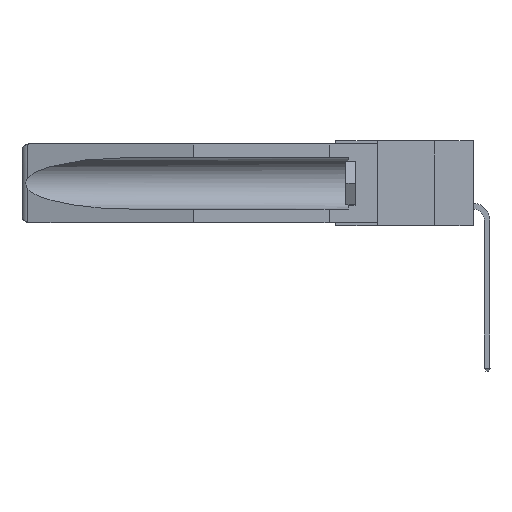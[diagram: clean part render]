
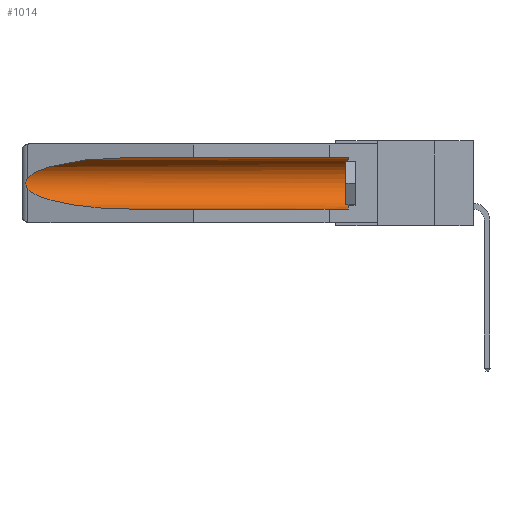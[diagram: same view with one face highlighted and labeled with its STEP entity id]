
A CAD part, left-side view. The second image highlights one B-rep face of the part: STEP entity #1014.
In plain terms, the highlighted cylindrical face has radius 2.857 mm (diameter 5.715 mm), a partial arc.
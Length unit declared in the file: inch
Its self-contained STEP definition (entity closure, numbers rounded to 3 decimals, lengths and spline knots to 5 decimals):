
#1 = EDGE_CURVE ( 'NONE', #16798, #9461, #5213, .T. ) ;
#342 = EDGE_CURVE ( 'NONE', #28409, #3035, #25971, .T. ) ;
#421 = CARTESIAN_POINT ( 'NONE',  ( 0.26597, 1.52961, -0.15275 ) ) ;
#663 = CARTESIAN_POINT ( 'NONE',  ( 0.155, -0.30754, -0.284 ) ) ;
#749 = CARTESIAN_POINT ( 'NONE',  ( 0.26655, 1.53094, -0.18657 ) ) ;
#1014 = ADVANCED_FACE ( 'NONE', ( #7717 ), #3617, .F. ) ;
#2842 = VERTEX_POINT ( 'NONE', #23426 ) ;
#3035 = VERTEX_POINT ( 'NONE', #10292 ) ;
#3096 = DIRECTION ( 'NONE',  ( 0., 1., 0. ) ) ;
#3443 = CARTESIAN_POINT ( 'NONE',  ( 0.155, 0.126, -0.1715 ) ) ;
#3617 = CYLINDRICAL_SURFACE ( 'NONE', #13320, 0.1125 ) ;
#3730 = VERTEX_POINT ( 'NONE', #18073 ) ;
#3817 = CARTESIAN_POINT ( 'NONE',  ( 0.155, 1.07973, -0.284 ) ) ;
#4316 = CARTESIAN_POINT ( 'NONE',  ( 0.26537, 1.52718, -0.14972 ) ) ;
#4538 = CARTESIAN_POINT ( 'NONE',  ( 0.155, 1.07973, -0.284 ) ) ;
#4825 =( BOUNDED_CURVE ( )  B_SPLINE_CURVE ( 3, ( #25880, #23379, #13919, #4316 ),
 .UNSPECIFIED., .F., .F. ) 
 B_SPLINE_CURVE_WITH_KNOTS ( ( 4, 4 ),
 ( 4.71239, 6.08839 ),
 .UNSPECIFIED. ) 
 CURVE ( )  GEOMETRIC_REPRESENTATION_ITEM ( )  RATIONAL_B_SPLINE_CURVE ( ( 1., 0.848, 0.848, 1. ) ) 
 REPRESENTATION_ITEM ( '' )  );
#5213 = LINE ( 'NONE', #663, #25657 ) ;
#6228 = CIRCLE ( 'NONE', #29589, 0.1125 ) ;
#7695 = EDGE_LOOP ( 'NONE', ( #25274, #15216, #8039, #23399, #27184, #23420 ) ) ;
#7717 = FACE_OUTER_BOUND ( 'NONE', #7695, .T. ) ;
#8039 = ORIENTED_EDGE ( 'NONE', *, *, #24191, .T. ) ;
#8237 = DIRECTION ( 'NONE',  ( 0., 0., 1. ) ) ;
#9395 = EDGE_CURVE ( 'NONE', #2842, #3730, #23835, .T. ) ;
#9461 = VERTEX_POINT ( 'NONE', #3817 ) ;
#10206 = CARTESIAN_POINT ( 'NONE',  ( 0.2675, 1.53308, -0.17534 ) ) ;
#10292 = CARTESIAN_POINT ( 'NONE',  ( 0.155, 1.07973, -0.059 ) ) ;
#10418 = CARTESIAN_POINT ( 'NONE',  ( 0.26597, 1.5296, -0.19026 ) ) ;
#10923 = CARTESIAN_POINT ( 'NONE',  ( 0.26537, 1.52718, -0.19328 ) ) ;
#11360 = CARTESIAN_POINT ( 'NONE',  ( 0.155, -0.30754, -0.059 ) ) ;
#12404 = CARTESIAN_POINT ( 'NONE',  ( 0.2673, 1.5327, -0.16383 ) ) ;
#12619 = CARTESIAN_POINT ( 'NONE',  ( 0.2673, 1.53269, -0.17917 ) ) ;
#13152 = DIRECTION ( 'NONE',  ( 0., 1., 0. ) ) ;
#13320 = AXIS2_PLACEMENT_3D ( 'NONE', #30011, #13152, #15746 ) ;
#13706 = VECTOR ( 'NONE', #20822, 39.37008 ) ;
#13919 = CARTESIAN_POINT ( 'NONE',  ( 0.25451, 1.48313, -0.09465 ) ) ;
#15216 = ORIENTED_EDGE ( 'NONE', *, *, #9395, .T. ) ;
#15746 = DIRECTION ( 'NONE',  ( 0., 0., 1. ) ) ;
#16798 = VERTEX_POINT ( 'NONE', #28485 ) ;
#17051 = CARTESIAN_POINT ( 'NONE',  ( 0.26654, 1.53092, -0.15636 ) ) ;
#18073 = CARTESIAN_POINT ( 'NONE',  ( 0.26537, 1.52718, -0.19328 ) ) ;
#18479 = CARTESIAN_POINT ( 'NONE',  ( 0.21114, 1.30732, -0.284 ) ) ;
#19547 = CARTESIAN_POINT ( 'NONE',  ( 0.2675, 1.53308, -0.16763 ) ) ;
#20068 = EDGE_CURVE ( 'NONE', #16798, #28409, #6228, .T. ) ;
#20822 = DIRECTION ( 'NONE',  ( 0., 1., 0. ) ) ;
#21731 = CARTESIAN_POINT ( 'NONE',  ( 0.26537, 1.52718, -0.14972 ) ) ;
#22924 = CARTESIAN_POINT ( 'NONE',  ( 0.155, 0.126, -0.059 ) ) ;
#23379 = CARTESIAN_POINT ( 'NONE',  ( 0.21114, 1.30732, -0.059 ) ) ;
#23399 = ORIENTED_EDGE ( 'NONE', *, *, #1, .F. ) ;
#23420 = ORIENTED_EDGE ( 'NONE', *, *, #342, .T. ) ;
#23426 = CARTESIAN_POINT ( 'NONE',  ( 0.26537, 1.52718, -0.14972 ) ) ;
#23835 = B_SPLINE_CURVE_WITH_KNOTS ( 'NONE', 3,
 ( #21731, #421, #17051, #12404, #19547, #10206, #12619, #749, #10418, #26963 ),
 .UNSPECIFIED., .F., .F.,
 ( 4, 2, 2, 2, 4 ),
 ( 0., 0.00029, 0.00058, 0.00087, 0.00117 ),
 .UNSPECIFIED. ) ;
#24191 = EDGE_CURVE ( 'NONE', #3730, #9461, #26496, .T. ) ;
#25078 = EDGE_CURVE ( 'NONE', #3035, #2842, #4825, .T. ) ;
#25274 = ORIENTED_EDGE ( 'NONE', *, *, #25078, .T. ) ;
#25657 = VECTOR ( 'NONE', #3096, 39.37008 ) ;
#25880 = CARTESIAN_POINT ( 'NONE',  ( 0.155, 1.07973, -0.059 ) ) ;
#25971 = LINE ( 'NONE', #11360, #13706 ) ;
#26496 =( BOUNDED_CURVE ( )  B_SPLINE_CURVE ( 3, ( #10923, #27582, #18479, #4538 ),
 .UNSPECIFIED., .F., .F. ) 
 B_SPLINE_CURVE_WITH_KNOTS ( ( 4, 4 ),
 ( 0.1948, 1.5708 ),
 .UNSPECIFIED. ) 
 CURVE ( )  GEOMETRIC_REPRESENTATION_ITEM ( )  RATIONAL_B_SPLINE_CURVE ( ( 1., 0.848, 0.848, 1. ) ) 
 REPRESENTATION_ITEM ( '' )  );
#26963 = CARTESIAN_POINT ( 'NONE',  ( 0.26537, 1.52718, -0.19328 ) ) ;
#27184 = ORIENTED_EDGE ( 'NONE', *, *, #20068, .T. ) ;
#27582 = CARTESIAN_POINT ( 'NONE',  ( 0.25451, 1.48313, -0.24835 ) ) ;
#28409 = VERTEX_POINT ( 'NONE', #22924 ) ;
#28485 = CARTESIAN_POINT ( 'NONE',  ( 0.155, 0.126, -0.284 ) ) ;
#29589 = AXIS2_PLACEMENT_3D ( 'NONE', #3443, #29737, #8237 ) ;
#29737 = DIRECTION ( 'NONE',  ( 0., -1., 0. ) ) ;
#30011 = CARTESIAN_POINT ( 'NONE',  ( 0.155, -0.30754, -0.1715 ) ) ;
